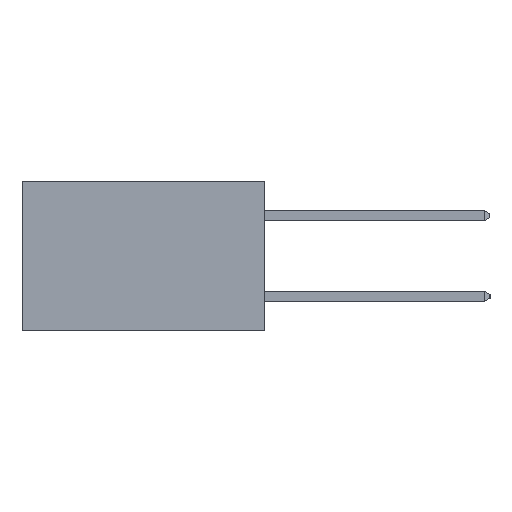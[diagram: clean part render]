
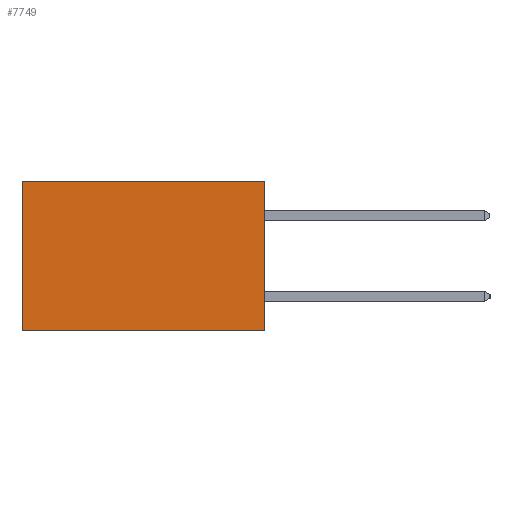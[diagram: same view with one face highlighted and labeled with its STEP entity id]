
A CAD part, left-side view. The second image highlights one B-rep face of the part: STEP entity #7749.
In plain terms, the highlighted planar face has unit normal (-1, 0, 0).
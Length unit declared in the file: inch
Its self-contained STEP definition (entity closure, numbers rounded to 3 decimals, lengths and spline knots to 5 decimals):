
#967 = VECTOR ( 'NONE', #11371, 39.37008 ) ;
#1031 = EDGE_CURVE ( 'NONE', #3818, #9657, #2454, .T. ) ;
#1836 = ORIENTED_EDGE ( 'NONE', *, *, #11112, .F. ) ;
#1907 = DIRECTION ( 'NONE',  ( 0., 0., -1. ) ) ;
#1985 = CARTESIAN_POINT ( 'NONE',  ( 0.2615, 0., 0. ) ) ;
#2154 = ORIENTED_EDGE ( 'NONE', *, *, #1031, .F. ) ;
#2454 = LINE ( 'NONE', #5734, #6990 ) ;
#2766 = ORIENTED_EDGE ( 'NONE', *, *, #4773, .T. ) ;
#2858 = CARTESIAN_POINT ( 'NONE',  ( 0.2615, 0.6, -0.37 ) ) ;
#2859 = LINE ( 'NONE', #9413, #5081 ) ;
#3223 = AXIS2_PLACEMENT_3D ( 'NONE', #10185, #9927, #9915 ) ;
#3349 = CARTESIAN_POINT ( 'NONE',  ( 0.2615, 0., -0.37 ) ) ;
#3777 = ORIENTED_EDGE ( 'NONE', *, *, #6647, .T. ) ;
#3818 = VERTEX_POINT ( 'NONE', #1985 ) ;
#4440 = EDGE_LOOP ( 'NONE', ( #3777, #1836, #2154, #2766 ) ) ;
#4511 = DIRECTION ( 'NONE',  ( 0., 1., 0. ) ) ;
#4773 = EDGE_CURVE ( 'NONE', #3818, #9578, #5500, .T. ) ;
#4824 = LINE ( 'NONE', #2858, #7465 ) ;
#4881 = CARTESIAN_POINT ( 'NONE',  ( 0.2615, 0.6, 0. ) ) ;
#5081 = VECTOR ( 'NONE', #4511, 39.37008 ) ;
#5281 = FACE_OUTER_BOUND ( 'NONE', #4440, .T. ) ;
#5500 = LINE ( 'NONE', #11472, #967 ) ;
#5734 = CARTESIAN_POINT ( 'NONE',  ( 0.2615, 0., -0.37 ) ) ;
#6071 = CARTESIAN_POINT ( 'NONE',  ( 0.2615, 0.6, -0.37 ) ) ;
#6647 = EDGE_CURVE ( 'NONE', #9578, #8013, #4824, .T. ) ;
#6792 = DIRECTION ( 'NONE',  ( 0., 0., -1. ) ) ;
#6990 = VECTOR ( 'NONE', #6792, 39.37008 ) ;
#7465 = VECTOR ( 'NONE', #1907, 39.37008 ) ;
#7749 = ADVANCED_FACE ( 'NONE', ( #5281 ), #9930, .F. ) ;
#8013 = VERTEX_POINT ( 'NONE', #6071 ) ;
#9413 = CARTESIAN_POINT ( 'NONE',  ( 0.2615, 0., -0.37 ) ) ;
#9578 = VERTEX_POINT ( 'NONE', #4881 ) ;
#9657 = VERTEX_POINT ( 'NONE', #3349 ) ;
#9915 = DIRECTION ( 'NONE',  ( 0., 0., -1. ) ) ;
#9927 = DIRECTION ( 'NONE',  ( 1., 0., 0. ) ) ;
#9930 = PLANE ( 'NONE',  #3223 ) ;
#10185 = CARTESIAN_POINT ( 'NONE',  ( 0.2615, 0., -0.37 ) ) ;
#11112 = EDGE_CURVE ( 'NONE', #9657, #8013, #2859, .T. ) ;
#11371 = DIRECTION ( 'NONE',  ( 0., 1., 0. ) ) ;
#11472 = CARTESIAN_POINT ( 'NONE',  ( 0.2615, 0., 0. ) ) ;
